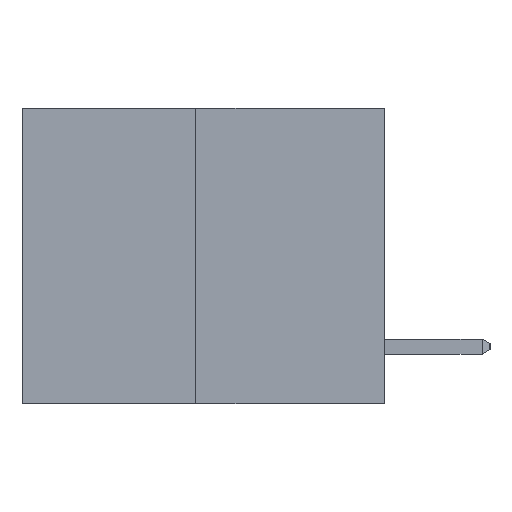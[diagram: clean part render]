
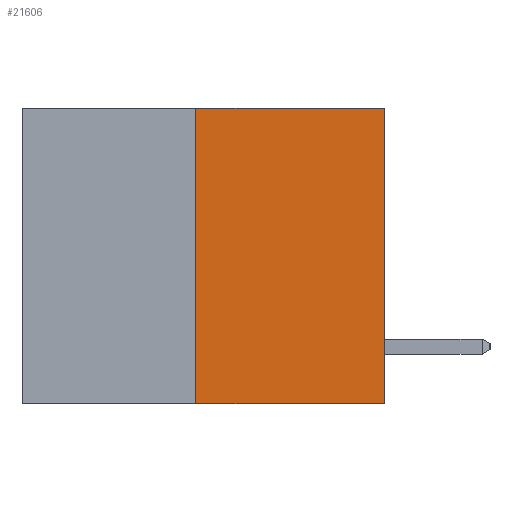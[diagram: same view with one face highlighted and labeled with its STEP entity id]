
A CAD part, left-side view. The second image highlights one B-rep face of the part: STEP entity #21606.
In plain terms, the highlighted planar face has unit normal (-1, 0, 0).
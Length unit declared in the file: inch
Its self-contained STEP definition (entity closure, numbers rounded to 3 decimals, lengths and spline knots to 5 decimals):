
#821 = DIRECTION ( 'NONE',  ( 0., 0., 1. ) ) ;
#860 = CARTESIAN_POINT ( 'NONE',  ( 0., 0.6, -0.49 ) ) ;
#1355 = EDGE_CURVE ( 'NONE', #3698, #28541, #8771, .T. ) ;
#3095 = EDGE_CURVE ( 'NONE', #8693, #4180, #24491, .T. ) ;
#3195 = PLANE ( 'NONE',  #21571 ) ;
#3202 = ORIENTED_EDGE ( 'NONE', *, *, #3095, .T. ) ;
#3698 = VERTEX_POINT ( 'NONE', #18720 ) ;
#4180 = VERTEX_POINT ( 'NONE', #29018 ) ;
#4867 = DIRECTION ( 'NONE',  ( 0., 0., 1. ) ) ;
#5360 = EDGE_LOOP ( 'NONE', ( #21017, #3202, #21244, #15321 ) ) ;
#5496 = VECTOR ( 'NONE', #7478, 39.37008 ) ;
#5771 = EDGE_CURVE ( 'NONE', #4180, #28541, #13101, .T. ) ;
#7478 = DIRECTION ( 'NONE',  ( 0., -1., 0. ) ) ;
#7608 = CARTESIAN_POINT ( 'NONE',  ( 0., 0.312, -0.49 ) ) ;
#8693 = VERTEX_POINT ( 'NONE', #7608 ) ;
#8771 = LINE ( 'NONE', #28217, #5496 ) ;
#10390 = DIRECTION ( 'NONE',  ( 0., -1., 0. ) ) ;
#12260 = CARTESIAN_POINT ( 'NONE',  ( 0., 0.312, -0.49 ) ) ;
#12371 = DIRECTION ( 'NONE',  ( 0., 0., -1. ) ) ;
#13101 = LINE ( 'NONE', #18864, #16008 ) ;
#15321 = ORIENTED_EDGE ( 'NONE', *, *, #1355, .F. ) ;
#15865 = VECTOR ( 'NONE', #821, 39.37008 ) ;
#16008 = VECTOR ( 'NONE', #4867, 39.37008 ) ;
#17092 = CARTESIAN_POINT ( 'NONE',  ( 0., 0.6, 0. ) ) ;
#17395 = EDGE_CURVE ( 'NONE', #8693, #3698, #22701, .T. ) ;
#18163 = CARTESIAN_POINT ( 'NONE',  ( 0., 0., 0. ) ) ;
#18720 = CARTESIAN_POINT ( 'NONE',  ( 0., 0.312, 0. ) ) ;
#18864 = CARTESIAN_POINT ( 'NONE',  ( 0., 0., 0. ) ) ;
#20951 = FACE_OUTER_BOUND ( 'NONE', #5360, .T. ) ;
#21017 = ORIENTED_EDGE ( 'NONE', *, *, #17395, .F. ) ;
#21244 = ORIENTED_EDGE ( 'NONE', *, *, #5771, .T. ) ;
#21571 = AXIS2_PLACEMENT_3D ( 'NONE', #17092, #23745, #12371 ) ;
#21606 = ADVANCED_FACE ( 'NONE', ( #20951 ), #3195, .F. ) ;
#22701 = LINE ( 'NONE', #12260, #15865 ) ;
#23745 = DIRECTION ( 'NONE',  ( 1., 0., 0. ) ) ;
#24491 = LINE ( 'NONE', #860, #25184 ) ;
#25184 = VECTOR ( 'NONE', #10390, 39.37008 ) ;
#28217 = CARTESIAN_POINT ( 'NONE',  ( 0., 0.6, 0. ) ) ;
#28541 = VERTEX_POINT ( 'NONE', #18163 ) ;
#29018 = CARTESIAN_POINT ( 'NONE',  ( 0., 0., -0.49 ) ) ;
